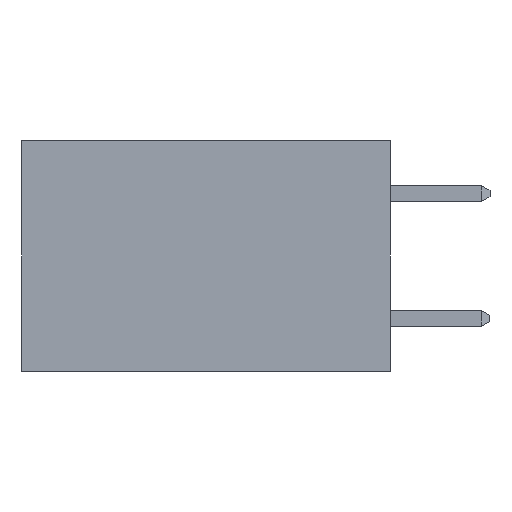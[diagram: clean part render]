
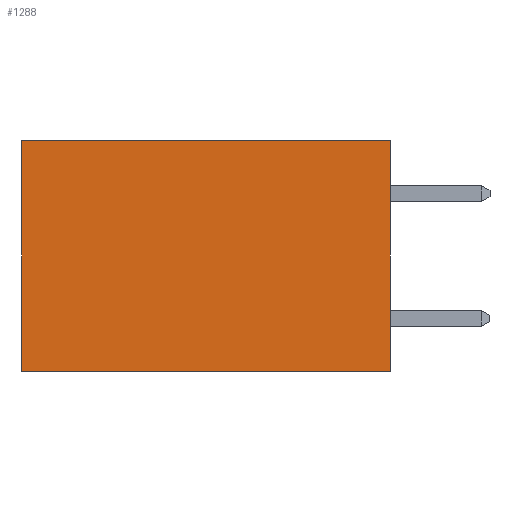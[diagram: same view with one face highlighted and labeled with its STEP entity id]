
A CAD part, left-side view. The second image highlights one B-rep face of the part: STEP entity #1288.
In plain terms, the highlighted planar face has unit normal (-1, 0, 0).
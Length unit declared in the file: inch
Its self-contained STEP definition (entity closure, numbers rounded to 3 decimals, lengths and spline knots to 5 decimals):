
#702 = CARTESIAN_POINT ( 'NONE',  ( 0.277, 0., -0.37 ) ) ;
#791 = DIRECTION ( 'NONE',  ( 0., 1., 0. ) ) ;
#807 = VECTOR ( 'NONE', #4833, 39.37008 ) ;
#1049 = VERTEX_POINT ( 'NONE', #7952 ) ;
#1288 = ADVANCED_FACE ( 'NONE', ( #4646 ), #4187, .F. ) ;
#1464 = LINE ( 'NONE', #702, #6396 ) ;
#1569 = VECTOR ( 'NONE', #3633, 39.37008 ) ;
#1921 = VERTEX_POINT ( 'NONE', #7561 ) ;
#2122 = VECTOR ( 'NONE', #6366, 39.37008 ) ;
#2322 = ORIENTED_EDGE ( 'NONE', *, *, #3532, .T. ) ;
#2447 = VERTEX_POINT ( 'NONE', #7302 ) ;
#2451 = ORIENTED_EDGE ( 'NONE', *, *, #3426, .F. ) ;
#2619 = ORIENTED_EDGE ( 'NONE', *, *, #3643, .F. ) ;
#2753 = ORIENTED_EDGE ( 'NONE', *, *, #3313, .T. ) ;
#2868 = LINE ( 'NONE', #5090, #807 ) ;
#3080 = EDGE_LOOP ( 'NONE', ( #2753, #2619, #2451, #2322 ) ) ;
#3184 = LINE ( 'NONE', #3539, #1569 ) ;
#3313 = EDGE_CURVE ( 'NONE', #1049, #2447, #7230, .T. ) ;
#3426 = EDGE_CURVE ( 'NONE', #4423, #1921, #2868, .T. ) ;
#3532 = EDGE_CURVE ( 'NONE', #4423, #1049, #3184, .T. ) ;
#3539 = CARTESIAN_POINT ( 'NONE',  ( 0.277, 0., 0. ) ) ;
#3633 = DIRECTION ( 'NONE',  ( 0., 1., 0. ) ) ;
#3643 = EDGE_CURVE ( 'NONE', #1921, #2447, #1464, .T. ) ;
#4187 = PLANE ( 'NONE',  #4818 ) ;
#4423 = VERTEX_POINT ( 'NONE', #4630 ) ;
#4630 = CARTESIAN_POINT ( 'NONE',  ( 0.277, 0., 0. ) ) ;
#4646 = FACE_OUTER_BOUND ( 'NONE', #3080, .T. ) ;
#4818 = AXIS2_PLACEMENT_3D ( 'NONE', #6125, #6319, #6179 ) ;
#4833 = DIRECTION ( 'NONE',  ( 0., 0., -1. ) ) ;
#5090 = CARTESIAN_POINT ( 'NONE',  ( 0.277, 0., -0.37 ) ) ;
#6125 = CARTESIAN_POINT ( 'NONE',  ( 0.277, 0., -0.37 ) ) ;
#6179 = DIRECTION ( 'NONE',  ( 0., 0., -1. ) ) ;
#6273 = CARTESIAN_POINT ( 'NONE',  ( 0.277, 0.59, -0.37 ) ) ;
#6319 = DIRECTION ( 'NONE',  ( 1., 0., 0. ) ) ;
#6366 = DIRECTION ( 'NONE',  ( 0., 0., -1. ) ) ;
#6396 = VECTOR ( 'NONE', #791, 39.37008 ) ;
#7230 = LINE ( 'NONE', #6273, #2122 ) ;
#7302 = CARTESIAN_POINT ( 'NONE',  ( 0.277, 0.59, -0.37 ) ) ;
#7561 = CARTESIAN_POINT ( 'NONE',  ( 0.277, 0., -0.37 ) ) ;
#7952 = CARTESIAN_POINT ( 'NONE',  ( 0.277, 0.59, 0. ) ) ;
